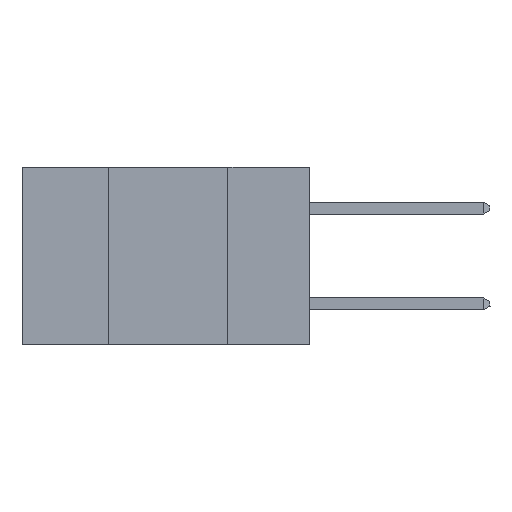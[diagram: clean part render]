
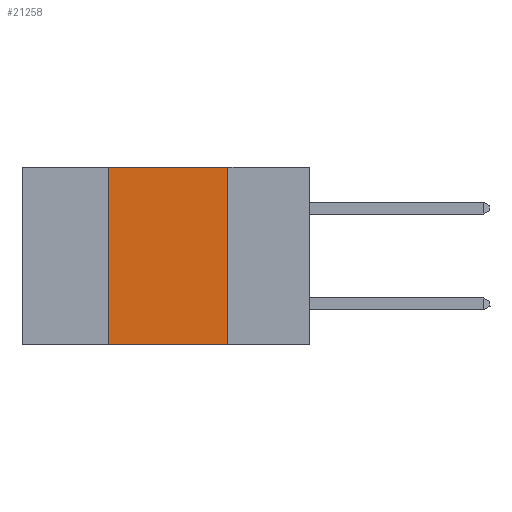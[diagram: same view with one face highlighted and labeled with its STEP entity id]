
A CAD part, left-side view. The second image highlights one B-rep face of the part: STEP entity #21258.
In plain terms, the highlighted planar face has unit normal (-1, 0, 0).
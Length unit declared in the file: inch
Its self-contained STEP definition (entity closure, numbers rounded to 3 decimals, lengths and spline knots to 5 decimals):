
#2542 = CARTESIAN_POINT ( 'NONE',  ( 0., 0.6, 0. ) ) ;
#6157 = VECTOR ( 'NONE', #34238, 39.37008 ) ;
#6490 = EDGE_CURVE ( 'NONE', #19944, #37136, #18244, .T. ) ;
#7720 = ORIENTED_EDGE ( 'NONE', *, *, #15891, .T. ) ;
#7962 = LINE ( 'NONE', #34694, #35203 ) ;
#10652 = VECTOR ( 'NONE', #18618, 39.37008 ) ;
#10943 = LINE ( 'NONE', #13796, #21773 ) ;
#11874 = EDGE_LOOP ( 'NONE', ( #28232, #30292, #20589, #7720 ) ) ;
#13298 = CARTESIAN_POINT ( 'NONE',  ( 0., 0.6, 0. ) ) ;
#13670 = EDGE_CURVE ( 'NONE', #37377, #19944, #10943, .T. ) ;
#13676 = CARTESIAN_POINT ( 'NONE',  ( 0., 0.42, -0.37 ) ) ;
#13796 = CARTESIAN_POINT ( 'NONE',  ( 0., 0.42, 0. ) ) ;
#14113 = DIRECTION ( 'NONE',  ( 0., 0., -1. ) ) ;
#15891 = EDGE_CURVE ( 'NONE', #37377, #20098, #7962, .T. ) ;
#16815 = EDGE_CURVE ( 'NONE', #37136, #20098, #19466, .T. ) ;
#18244 = LINE ( 'NONE', #13298, #10652 ) ;
#18267 = CARTESIAN_POINT ( 'NONE',  ( 0., 0.17, -0.37 ) ) ;
#18618 = DIRECTION ( 'NONE',  ( 0., -1., 0. ) ) ;
#19466 = LINE ( 'NONE', #22303, #6157 ) ;
#19944 = VERTEX_POINT ( 'NONE', #23202 ) ;
#20098 = VERTEX_POINT ( 'NONE', #18267 ) ;
#20589 = ORIENTED_EDGE ( 'NONE', *, *, #13670, .F. ) ;
#21258 = ADVANCED_FACE ( 'NONE', ( #23017 ), #28541, .F. ) ;
#21773 = VECTOR ( 'NONE', #28212, 39.37008 ) ;
#22303 = CARTESIAN_POINT ( 'NONE',  ( 0., 0.17, 0. ) ) ;
#22947 = DIRECTION ( 'NONE',  ( 0., -1., 0. ) ) ;
#23017 = FACE_OUTER_BOUND ( 'NONE', #11874, .T. ) ;
#23202 = CARTESIAN_POINT ( 'NONE',  ( 0., 0.42, 0. ) ) ;
#28212 = DIRECTION ( 'NONE',  ( 0., 0., 1. ) ) ;
#28232 = ORIENTED_EDGE ( 'NONE', *, *, #16815, .F. ) ;
#28541 = PLANE ( 'NONE',  #30527 ) ;
#28721 = DIRECTION ( 'NONE',  ( 1., 0., 0. ) ) ;
#30292 = ORIENTED_EDGE ( 'NONE', *, *, #6490, .F. ) ;
#30527 = AXIS2_PLACEMENT_3D ( 'NONE', #2542, #28721, #14113 ) ;
#34238 = DIRECTION ( 'NONE',  ( 0., 0., -1. ) ) ;
#34694 = CARTESIAN_POINT ( 'NONE',  ( 0., 0.6, -0.37 ) ) ;
#35203 = VECTOR ( 'NONE', #22947, 39.37008 ) ;
#37136 = VERTEX_POINT ( 'NONE', #37400 ) ;
#37377 = VERTEX_POINT ( 'NONE', #13676 ) ;
#37400 = CARTESIAN_POINT ( 'NONE',  ( 0., 0.17, 0. ) ) ;
